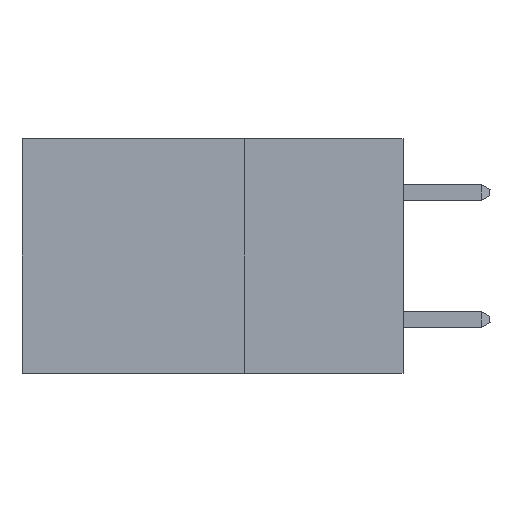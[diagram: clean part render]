
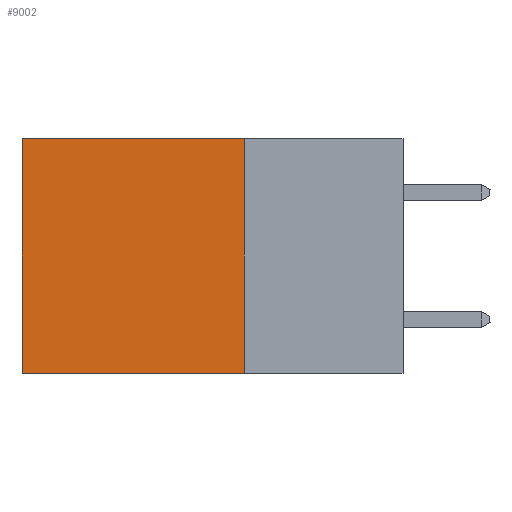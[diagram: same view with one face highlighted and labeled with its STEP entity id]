
A CAD part, left-side view. The second image highlights one B-rep face of the part: STEP entity #9002.
In plain terms, the highlighted planar face has unit normal (-1, 0, 0).
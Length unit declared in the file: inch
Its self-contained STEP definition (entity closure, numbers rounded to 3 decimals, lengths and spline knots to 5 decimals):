
#8 = LINE ( 'NONE', #16170, #6629 ) ;
#646 = CARTESIAN_POINT ( 'NONE',  ( 0.2875, 0.25, 0. ) ) ;
#1617 = DIRECTION ( 'NONE',  ( 1., 0., 0. ) ) ;
#2357 = CARTESIAN_POINT ( 'NONE',  ( 0.2875, 0.25, 0. ) ) ;
#3904 = LINE ( 'NONE', #12463, #11602 ) ;
#4202 = LINE ( 'NONE', #2357, #12776 ) ;
#5307 = DIRECTION ( 'NONE',  ( 0., 0., -1. ) ) ;
#5385 = CARTESIAN_POINT ( 'NONE',  ( 0.2875, 0.6, -0.37 ) ) ;
#6629 = VECTOR ( 'NONE', #9024, 39.37008 ) ;
#7163 = VERTEX_POINT ( 'NONE', #5385 ) ;
#7946 = DIRECTION ( 'NONE',  ( 0., 0., -1. ) ) ;
#8640 = EDGE_CURVE ( 'NONE', #13661, #11900, #4202, .T. ) ;
#8967 = LINE ( 'NONE', #646, #17314 ) ;
#9002 = ADVANCED_FACE ( 'NONE', ( #11053 ), #12731, .F. ) ;
#9024 = DIRECTION ( 'NONE',  ( 0., 1., 0. ) ) ;
#9586 = VERTEX_POINT ( 'NONE', #18455 ) ;
#9861 = DIRECTION ( 'NONE',  ( 0., 1., 0. ) ) ;
#10484 = CARTESIAN_POINT ( 'NONE',  ( 0.2875, 0.25, -0.37 ) ) ;
#11053 = FACE_OUTER_BOUND ( 'NONE', #11357, .T. ) ;
#11357 = EDGE_LOOP ( 'NONE', ( #20428, #15385, #18527, #14389 ) ) ;
#11602 = VECTOR ( 'NONE', #14321, 39.37008 ) ;
#11900 = VERTEX_POINT ( 'NONE', #10484 ) ;
#12463 = CARTESIAN_POINT ( 'NONE',  ( 0.2875, 0.6, 0. ) ) ;
#12562 = CARTESIAN_POINT ( 'NONE',  ( 0.2875, 0.25, 0. ) ) ;
#12731 = PLANE ( 'NONE',  #16019 ) ;
#12776 = VECTOR ( 'NONE', #7946, 39.37008 ) ;
#13661 = VERTEX_POINT ( 'NONE', #21793 ) ;
#13674 = EDGE_CURVE ( 'NONE', #11900, #7163, #8, .T. ) ;
#14321 = DIRECTION ( 'NONE',  ( 0., 0., -1. ) ) ;
#14389 = ORIENTED_EDGE ( 'NONE', *, *, #19533, .T. ) ;
#15385 = ORIENTED_EDGE ( 'NONE', *, *, #13674, .F. ) ;
#16019 = AXIS2_PLACEMENT_3D ( 'NONE', #12562, #1617, #5307 ) ;
#16170 = CARTESIAN_POINT ( 'NONE',  ( 0.2875, 0.25, -0.37 ) ) ;
#17314 = VECTOR ( 'NONE', #9861, 39.37008 ) ;
#17966 = EDGE_CURVE ( 'NONE', #9586, #7163, #3904, .T. ) ;
#18455 = CARTESIAN_POINT ( 'NONE',  ( 0.2875, 0.6, 0. ) ) ;
#18527 = ORIENTED_EDGE ( 'NONE', *, *, #8640, .F. ) ;
#19533 = EDGE_CURVE ( 'NONE', #13661, #9586, #8967, .T. ) ;
#20428 = ORIENTED_EDGE ( 'NONE', *, *, #17966, .T. ) ;
#21793 = CARTESIAN_POINT ( 'NONE',  ( 0.2875, 0.25, 0. ) ) ;
